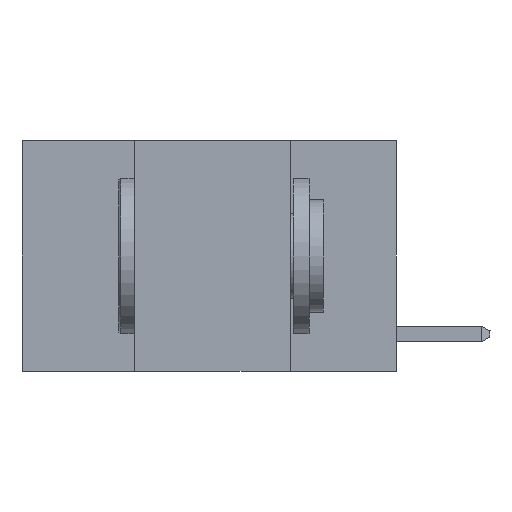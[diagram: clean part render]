
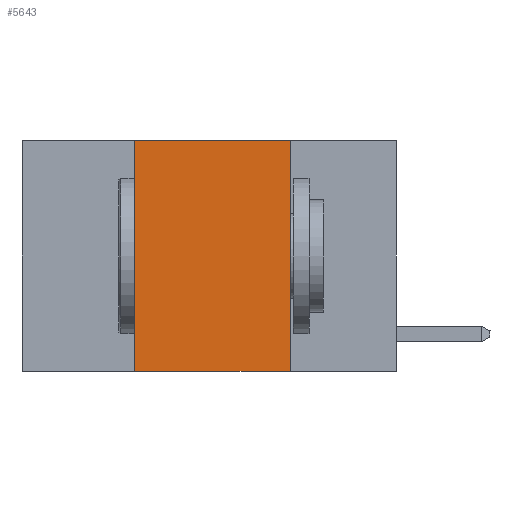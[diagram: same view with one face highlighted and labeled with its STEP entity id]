
A CAD part, left-side view. The second image highlights one B-rep face of the part: STEP entity #5643.
In plain terms, the highlighted planar face has unit normal (-1, 0, 0).
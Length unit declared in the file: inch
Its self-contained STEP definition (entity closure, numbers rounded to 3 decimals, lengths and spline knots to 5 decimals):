
#562 = DIRECTION ( 'NONE',  ( 1., 0., 0. ) ) ;
#900 = CARTESIAN_POINT ( 'NONE',  ( 0., 0.42, -0.37 ) ) ;
#1357 = DIRECTION ( 'NONE',  ( 0., -1., 0. ) ) ;
#1497 = ORIENTED_EDGE ( 'NONE', *, *, #7105, .F. ) ;
#3417 = EDGE_CURVE ( 'NONE', #10662, #6891, #12167, .T. ) ;
#4657 = DIRECTION ( 'NONE',  ( 0., 0., -1. ) ) ;
#5199 = CARTESIAN_POINT ( 'NONE',  ( 0., 0.6, 0. ) ) ;
#5643 = ADVANCED_FACE ( 'NONE', ( #11244 ), #14666, .F. ) ;
#5646 = CARTESIAN_POINT ( 'NONE',  ( 0., 0.17, 0. ) ) ;
#5748 = VERTEX_POINT ( 'NONE', #8995 ) ;
#5862 = EDGE_CURVE ( 'NONE', #6891, #8051, #12939, .T. ) ;
#6645 = ORIENTED_EDGE ( 'NONE', *, *, #5862, .F. ) ;
#6891 = VERTEX_POINT ( 'NONE', #7828 ) ;
#6894 = LINE ( 'NONE', #5646, #11843 ) ;
#7105 = EDGE_CURVE ( 'NONE', #8051, #5748, #6894, .T. ) ;
#7185 = ORIENTED_EDGE ( 'NONE', *, *, #10622, .T. ) ;
#7828 = CARTESIAN_POINT ( 'NONE',  ( 0., 0.42, 0. ) ) ;
#8051 = VERTEX_POINT ( 'NONE', #10113 ) ;
#8345 = CARTESIAN_POINT ( 'NONE',  ( 0., 0.6, 0. ) ) ;
#8452 = CARTESIAN_POINT ( 'NONE',  ( 0., 0.6, -0.37 ) ) ;
#8653 = DIRECTION ( 'NONE',  ( 0., 0., -1. ) ) ;
#8995 = CARTESIAN_POINT ( 'NONE',  ( 0., 0.17, -0.37 ) ) ;
#9564 = CARTESIAN_POINT ( 'NONE',  ( 0., 0.42, 0. ) ) ;
#10113 = CARTESIAN_POINT ( 'NONE',  ( 0., 0.17, 0. ) ) ;
#10569 = ORIENTED_EDGE ( 'NONE', *, *, #3417, .F. ) ;
#10622 = EDGE_CURVE ( 'NONE', #10662, #5748, #12389, .T. ) ;
#10662 = VERTEX_POINT ( 'NONE', #900 ) ;
#11244 = FACE_OUTER_BOUND ( 'NONE', #13688, .T. ) ;
#11843 = VECTOR ( 'NONE', #4657, 39.37008 ) ;
#12167 = LINE ( 'NONE', #9564, #16608 ) ;
#12389 = LINE ( 'NONE', #8452, #14052 ) ;
#12939 = LINE ( 'NONE', #5199, #16395 ) ;
#13165 = AXIS2_PLACEMENT_3D ( 'NONE', #8345, #562, #8653 ) ;
#13688 = EDGE_LOOP ( 'NONE', ( #1497, #6645, #10569, #7185 ) ) ;
#13758 = DIRECTION ( 'NONE',  ( 0., 0., 1. ) ) ;
#14052 = VECTOR ( 'NONE', #14851, 39.37008 ) ;
#14666 = PLANE ( 'NONE',  #13165 ) ;
#14851 = DIRECTION ( 'NONE',  ( 0., -1., 0. ) ) ;
#16395 = VECTOR ( 'NONE', #1357, 39.37008 ) ;
#16608 = VECTOR ( 'NONE', #13758, 39.37008 ) ;
